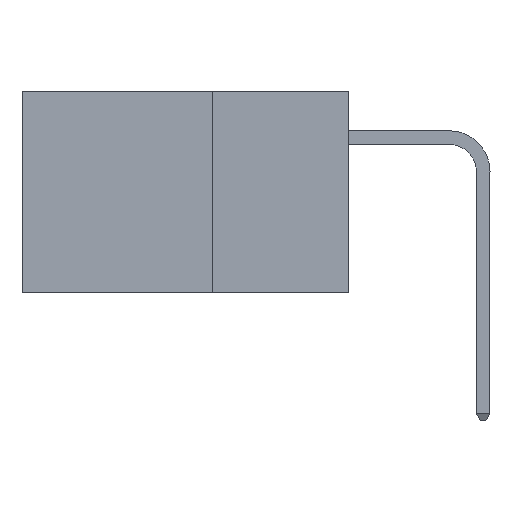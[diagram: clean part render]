
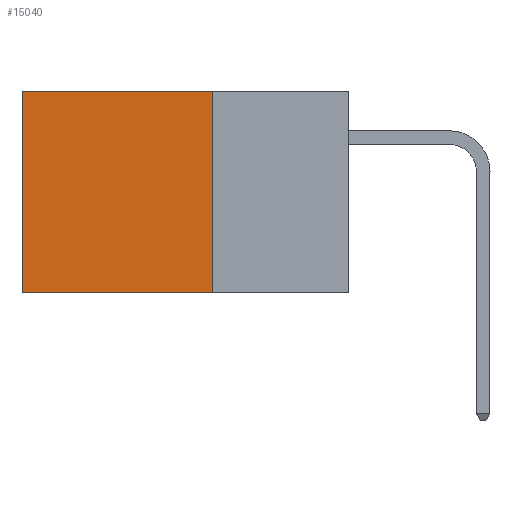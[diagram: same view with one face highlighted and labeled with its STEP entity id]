
A CAD part, left-side view. The second image highlights one B-rep face of the part: STEP entity #15040.
In plain terms, the highlighted planar face has unit normal (-1, 0, 0).
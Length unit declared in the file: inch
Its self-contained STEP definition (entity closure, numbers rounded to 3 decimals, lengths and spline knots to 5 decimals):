
#125 = CARTESIAN_POINT ( 'NONE',  ( 0.2875, 0.25, 0. ) ) ;
#287 = LINE ( 'NONE', #15159, #5191 ) ;
#320 = LINE ( 'NONE', #125, #22283 ) ;
#1364 = DIRECTION ( 'NONE',  ( 0., 1., 0. ) ) ;
#1452 = AXIS2_PLACEMENT_3D ( 'NONE', #11663, #9932, #22680 ) ;
#2828 = CARTESIAN_POINT ( 'NONE',  ( 0.2875, 0.25, -0.37 ) ) ;
#3317 = VERTEX_POINT ( 'NONE', #2828 ) ;
#4172 = VERTEX_POINT ( 'NONE', #7051 ) ;
#4490 = CARTESIAN_POINT ( 'NONE',  ( 0.2875, 0.6, 0. ) ) ;
#4997 = VERTEX_POINT ( 'NONE', #16446 ) ;
#5133 = VECTOR ( 'NONE', #20620, 39.37008 ) ;
#5191 = VECTOR ( 'NONE', #17496, 39.37008 ) ;
#5723 = PLANE ( 'NONE',  #1452 ) ;
#6279 = EDGE_CURVE ( 'NONE', #4172, #3317, #320, .T. ) ;
#7051 = CARTESIAN_POINT ( 'NONE',  ( 0.2875, 0.25, 0. ) ) ;
#7215 = VECTOR ( 'NONE', #1364, 39.37008 ) ;
#7693 = EDGE_LOOP ( 'NONE', ( #21229, #12708, #23342, #11035 ) ) ;
#9932 = DIRECTION ( 'NONE',  ( 1., 0., 0. ) ) ;
#11035 = ORIENTED_EDGE ( 'NONE', *, *, #19583, .T. ) ;
#11663 = CARTESIAN_POINT ( 'NONE',  ( 0.2875, 0.25, 0. ) ) ;
#12069 = LINE ( 'NONE', #12164, #7215 ) ;
#12164 = CARTESIAN_POINT ( 'NONE',  ( 0.2875, 0.25, 0. ) ) ;
#12708 = ORIENTED_EDGE ( 'NONE', *, *, #21503, .F. ) ;
#15040 = ADVANCED_FACE ( 'NONE', ( #19416 ), #5723, .F. ) ;
#15159 = CARTESIAN_POINT ( 'NONE',  ( 0.2875, 0.25, -0.37 ) ) ;
#16208 = EDGE_CURVE ( 'NONE', #4997, #18714, #18771, .T. ) ;
#16446 = CARTESIAN_POINT ( 'NONE',  ( 0.2875, 0.6, 0. ) ) ;
#17496 = DIRECTION ( 'NONE',  ( 0., 1., 0. ) ) ;
#17855 = CARTESIAN_POINT ( 'NONE',  ( 0.2875, 0.6, -0.37 ) ) ;
#18714 = VERTEX_POINT ( 'NONE', #17855 ) ;
#18771 = LINE ( 'NONE', #4490, #5133 ) ;
#19416 = FACE_OUTER_BOUND ( 'NONE', #7693, .T. ) ;
#19583 = EDGE_CURVE ( 'NONE', #4172, #4997, #12069, .T. ) ;
#19983 = DIRECTION ( 'NONE',  ( 0., 0., -1. ) ) ;
#20620 = DIRECTION ( 'NONE',  ( 0., 0., -1. ) ) ;
#21229 = ORIENTED_EDGE ( 'NONE', *, *, #16208, .T. ) ;
#21503 = EDGE_CURVE ( 'NONE', #3317, #18714, #287, .T. ) ;
#22283 = VECTOR ( 'NONE', #19983, 39.37008 ) ;
#22680 = DIRECTION ( 'NONE',  ( 0., 0., -1. ) ) ;
#23342 = ORIENTED_EDGE ( 'NONE', *, *, #6279, .F. ) ;
